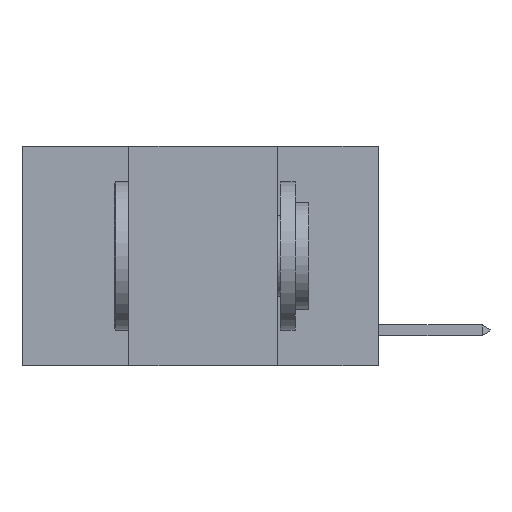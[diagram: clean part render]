
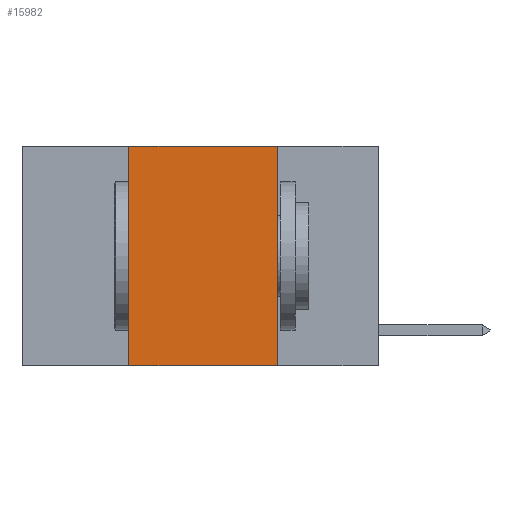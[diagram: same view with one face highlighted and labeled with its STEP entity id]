
A CAD part, left-side view. The second image highlights one B-rep face of the part: STEP entity #15982.
In plain terms, the highlighted planar face has unit normal (-1, 0, 0).
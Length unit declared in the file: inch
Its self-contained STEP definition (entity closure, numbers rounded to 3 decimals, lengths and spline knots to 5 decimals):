
#339 = LINE ( 'NONE', #2009, #18934 ) ;
#809 = VERTEX_POINT ( 'NONE', #17812 ) ;
#1685 = DIRECTION ( 'NONE',  ( 0., -1., 0. ) ) ;
#1840 = FACE_OUTER_BOUND ( 'NONE', #6681, .T. ) ;
#2009 = CARTESIAN_POINT ( 'NONE',  ( 0., 0.17, 0. ) ) ;
#2489 = CARTESIAN_POINT ( 'NONE',  ( 0., 0.42, 0. ) ) ;
#3027 = EDGE_CURVE ( 'NONE', #10046, #7784, #4615, .T. ) ;
#3193 = DIRECTION ( 'NONE',  ( 1., 0., 0. ) ) ;
#4152 = DIRECTION ( 'NONE',  ( 0., 0., 1. ) ) ;
#4615 = LINE ( 'NONE', #5955, #4824 ) ;
#4824 = VECTOR ( 'NONE', #12290, 39.37008 ) ;
#5955 = CARTESIAN_POINT ( 'NONE',  ( 0., 0.6, -0.37 ) ) ;
#6355 = EDGE_CURVE ( 'NONE', #12304, #7784, #339, .T. ) ;
#6681 = EDGE_LOOP ( 'NONE', ( #10630, #10017, #15443, #15836 ) ) ;
#6691 = DIRECTION ( 'NONE',  ( 0., 0., -1. ) ) ;
#6920 = EDGE_CURVE ( 'NONE', #10046, #809, #16737, .T. ) ;
#7784 = VERTEX_POINT ( 'NONE', #9392 ) ;
#9392 = CARTESIAN_POINT ( 'NONE',  ( 0., 0.17, -0.37 ) ) ;
#10017 = ORIENTED_EDGE ( 'NONE', *, *, #20478, .F. ) ;
#10046 = VERTEX_POINT ( 'NONE', #13148 ) ;
#10630 = ORIENTED_EDGE ( 'NONE', *, *, #6355, .F. ) ;
#10819 = LINE ( 'NONE', #17610, #17250 ) ;
#10821 = AXIS2_PLACEMENT_3D ( 'NONE', #19328, #3193, #15882 ) ;
#12290 = DIRECTION ( 'NONE',  ( 0., -1., 0. ) ) ;
#12304 = VERTEX_POINT ( 'NONE', #17936 ) ;
#12736 = PLANE ( 'NONE',  #10821 ) ;
#13148 = CARTESIAN_POINT ( 'NONE',  ( 0., 0.42, -0.37 ) ) ;
#15443 = ORIENTED_EDGE ( 'NONE', *, *, #6920, .F. ) ;
#15836 = ORIENTED_EDGE ( 'NONE', *, *, #3027, .T. ) ;
#15882 = DIRECTION ( 'NONE',  ( 0., 0., -1. ) ) ;
#15982 = ADVANCED_FACE ( 'NONE', ( #1840 ), #12736, .F. ) ;
#16737 = LINE ( 'NONE', #2489, #18377 ) ;
#17250 = VECTOR ( 'NONE', #1685, 39.37008 ) ;
#17610 = CARTESIAN_POINT ( 'NONE',  ( 0., 0.6, 0. ) ) ;
#17812 = CARTESIAN_POINT ( 'NONE',  ( 0., 0.42, 0. ) ) ;
#17936 = CARTESIAN_POINT ( 'NONE',  ( 0., 0.17, 0. ) ) ;
#18377 = VECTOR ( 'NONE', #4152, 39.37008 ) ;
#18934 = VECTOR ( 'NONE', #6691, 39.37008 ) ;
#19328 = CARTESIAN_POINT ( 'NONE',  ( 0., 0.6, 0. ) ) ;
#20478 = EDGE_CURVE ( 'NONE', #809, #12304, #10819, .T. ) ;
